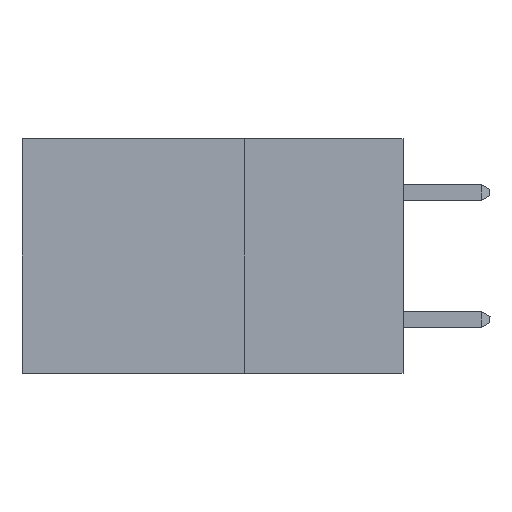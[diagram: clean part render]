
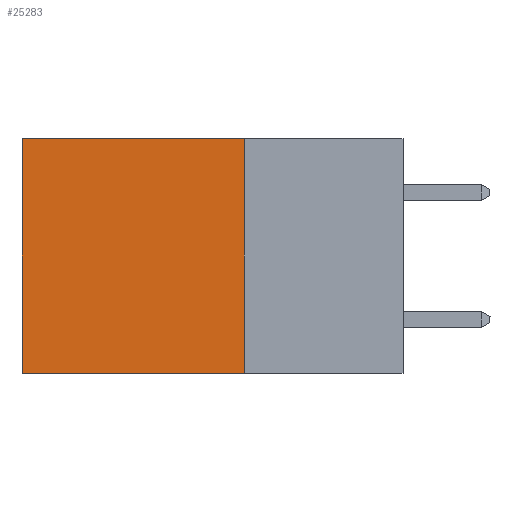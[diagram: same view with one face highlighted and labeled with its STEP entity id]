
A CAD part, left-side view. The second image highlights one B-rep face of the part: STEP entity #25283.
In plain terms, the highlighted planar face has unit normal (-1, 0, 0).
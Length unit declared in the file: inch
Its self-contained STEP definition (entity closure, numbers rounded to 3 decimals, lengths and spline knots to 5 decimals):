
#589 = VERTEX_POINT ( 'NONE', #10425 ) ;
#1697 = ORIENTED_EDGE ( 'NONE', *, *, #34432, .T. ) ;
#3230 = ORIENTED_EDGE ( 'NONE', *, *, #30824, .F. ) ;
#4505 = DIRECTION ( 'NONE',  ( 0., 1., 0. ) ) ;
#4574 = CARTESIAN_POINT ( 'NONE',  ( 0.2875, 0.6, -0.37 ) ) ;
#5107 = VECTOR ( 'NONE', #20435, 39.37008 ) ;
#5256 = LINE ( 'NONE', #21255, #31085 ) ;
#7809 = VECTOR ( 'NONE', #25512, 39.37008 ) ;
#8821 = VERTEX_POINT ( 'NONE', #16642 ) ;
#8851 = DIRECTION ( 'NONE',  ( 1., 0., 0. ) ) ;
#10404 = EDGE_CURVE ( 'NONE', #8821, #20498, #22682, .T. ) ;
#10425 = CARTESIAN_POINT ( 'NONE',  ( 0.2875, 0.25, -0.37 ) ) ;
#12027 = PLANE ( 'NONE',  #32233 ) ;
#12066 = FACE_OUTER_BOUND ( 'NONE', #42387, .T. ) ;
#16642 = CARTESIAN_POINT ( 'NONE',  ( 0.2875, 0.6, 0. ) ) ;
#16974 = VECTOR ( 'NONE', #40900, 39.37008 ) ;
#20435 = DIRECTION ( 'NONE',  ( 0., 0., -1. ) ) ;
#20498 = VERTEX_POINT ( 'NONE', #4574 ) ;
#21255 = CARTESIAN_POINT ( 'NONE',  ( 0.2875, 0.25, -0.37 ) ) ;
#22682 = LINE ( 'NONE', #24294, #5107 ) ;
#24294 = CARTESIAN_POINT ( 'NONE',  ( 0.2875, 0.6, 0. ) ) ;
#24554 = ORIENTED_EDGE ( 'NONE', *, *, #32907, .F. ) ;
#25283 = ADVANCED_FACE ( 'NONE', ( #12066 ), #12027, .F. ) ;
#25512 = DIRECTION ( 'NONE',  ( 0., 0., -1. ) ) ;
#25727 = CARTESIAN_POINT ( 'NONE',  ( 0.2875, 0.25, 0. ) ) ;
#26418 = LINE ( 'NONE', #42083, #7809 ) ;
#26489 = VERTEX_POINT ( 'NONE', #41696 ) ;
#27316 = LINE ( 'NONE', #37610, #16974 ) ;
#30824 = EDGE_CURVE ( 'NONE', #589, #20498, #5256, .T. ) ;
#31085 = VECTOR ( 'NONE', #4505, 39.37008 ) ;
#31900 = DIRECTION ( 'NONE',  ( 0., 0., -1. ) ) ;
#32233 = AXIS2_PLACEMENT_3D ( 'NONE', #25727, #8851, #31900 ) ;
#32907 = EDGE_CURVE ( 'NONE', #26489, #589, #26418, .T. ) ;
#33913 = ORIENTED_EDGE ( 'NONE', *, *, #10404, .T. ) ;
#34432 = EDGE_CURVE ( 'NONE', #26489, #8821, #27316, .T. ) ;
#37610 = CARTESIAN_POINT ( 'NONE',  ( 0.2875, 0.25, 0. ) ) ;
#40900 = DIRECTION ( 'NONE',  ( 0., 1., 0. ) ) ;
#41696 = CARTESIAN_POINT ( 'NONE',  ( 0.2875, 0.25, 0. ) ) ;
#42083 = CARTESIAN_POINT ( 'NONE',  ( 0.2875, 0.25, 0. ) ) ;
#42387 = EDGE_LOOP ( 'NONE', ( #33913, #3230, #24554, #1697 ) ) ;
